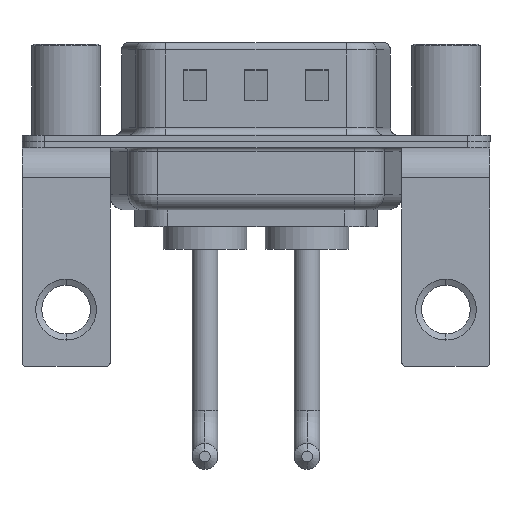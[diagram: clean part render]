
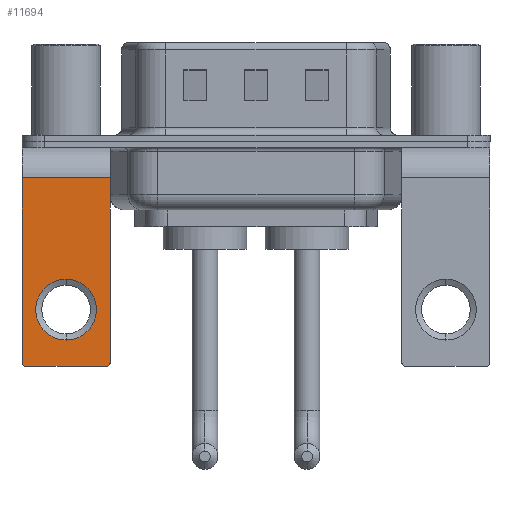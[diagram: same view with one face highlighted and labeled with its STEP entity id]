
A CAD part, front view. The second image highlights one B-rep face of the part: STEP entity #11694.
In plain terms, the highlighted planar face has unit normal (0, -1, 0).
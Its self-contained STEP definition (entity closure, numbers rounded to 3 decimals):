
#491 = EDGE_LOOP ( 'NONE', ( #12679, #11862, #15501, #12673, #6525, #12632 ) ) ;
#604 = EDGE_CURVE ( 'NONE', #1307, #2217, #11024, .T. ) ;
#1099 = CARTESIAN_POINT ( 'NONE',  ( 2.9, -6.25, -2.4 ) ) ;
#1121 = CARTESIAN_POINT ( 'NONE',  ( 0., -6.25, -9.07 ) ) ;
#1208 = VERTEX_POINT ( 'NONE', #5737 ) ;
#1215 = VECTOR ( 'NONE', #6323, 1000. ) ;
#1307 = VERTEX_POINT ( 'NONE', #8716 ) ;
#1532 = ORIENTED_EDGE ( 'NONE', *, *, #15060, .T. ) ;
#2217 = VERTEX_POINT ( 'NONE', #11225 ) ;
#2307 = DIRECTION ( 'NONE',  ( 0., -1., 0. ) ) ;
#2716 = CARTESIAN_POINT ( 'NONE',  ( -2.65, -6.25, -14.8 ) ) ;
#2738 = DIRECTION ( 'NONE',  ( 0., 0., -1. ) ) ;
#2911 = DIRECTION ( 'NONE',  ( 0., 1., 0. ) ) ;
#3023 = EDGE_CURVE ( 'NONE', #14362, #9159, #6748, .T. ) ;
#3037 = ORIENTED_EDGE ( 'NONE', *, *, #14663, .T. ) ;
#3417 = VERTEX_POINT ( 'NONE', #1099 ) ;
#4305 = VERTEX_POINT ( 'NONE', #1121 ) ;
#4631 = LINE ( 'NONE', #9841, #15808 ) ;
#4887 = DIRECTION ( 'NONE',  ( -1., 0., 0. ) ) ;
#4995 = EDGE_LOOP ( 'NONE', ( #1532, #3037 ) ) ;
#5540 = FACE_BOUND ( 'NONE', #4995, .T. ) ;
#5556 = DIRECTION ( 'NONE',  ( 0., 0., 1. ) ) ;
#5737 = CARTESIAN_POINT ( 'NONE',  ( 0., -6.25, -13.07 ) ) ;
#5770 = CARTESIAN_POINT ( 'NONE',  ( -2.9, -6.25, -14.55 ) ) ;
#5901 = CIRCLE ( 'NONE', #15966, 0.25 ) ;
#6263 = CARTESIAN_POINT ( 'NONE',  ( 2.9, -6.25, -2.4 ) ) ;
#6323 = DIRECTION ( 'NONE',  ( 0., 0., -1. ) ) ;
#6525 = ORIENTED_EDGE ( 'NONE', *, *, #15311, .F. ) ;
#6748 = LINE ( 'NONE', #10497, #16271 ) ;
#6910 = EDGE_CURVE ( 'NONE', #1307, #8998, #4631, .T. ) ;
#7039 = DIRECTION ( 'NONE',  ( -1., 0., 0. ) ) ;
#7084 = DIRECTION ( 'NONE',  ( 0., 0., 1. ) ) ;
#7998 = LINE ( 'NONE', #6263, #12092 ) ;
#8716 = CARTESIAN_POINT ( 'NONE',  ( 2.65, -6.25, -14.8 ) ) ;
#8728 = DIRECTION ( 'NONE',  ( 0., 0., 1. ) ) ;
#8998 = VERTEX_POINT ( 'NONE', #2716 ) ;
#9159 = VERTEX_POINT ( 'NONE', #5770 ) ;
#9306 = CARTESIAN_POINT ( 'NONE',  ( 0., -6.25, -11.07 ) ) ;
#9467 = DIRECTION ( 'NONE',  ( 0., 1., 0. ) ) ;
#9841 = CARTESIAN_POINT ( 'NONE',  ( 2.9, -6.25, -14.8 ) ) ;
#10257 = AXIS2_PLACEMENT_3D ( 'NONE', #9306, #2911, #5556 ) ;
#10497 = CARTESIAN_POINT ( 'NONE',  ( -2.9, -6.25, -2.4 ) ) ;
#10552 = CARTESIAN_POINT ( 'NONE',  ( 2.65, -6.25, -14.55 ) ) ;
#10735 = FACE_OUTER_BOUND ( 'NONE', #491, .T. ) ;
#10752 = AXIS2_PLACEMENT_3D ( 'NONE', #10552, #11033, #14782 ) ;
#11024 = CIRCLE ( 'NONE', #10752, 0.25 ) ;
#11033 = DIRECTION ( 'NONE',  ( 0., -1., 0. ) ) ;
#11225 = CARTESIAN_POINT ( 'NONE',  ( 2.9, -6.25, -14.55 ) ) ;
#11264 = CARTESIAN_POINT ( 'NONE',  ( -2.65, -6.25, -14.55 ) ) ;
#11368 = CARTESIAN_POINT ( 'NONE',  ( 0., -6.25, -11.07 ) ) ;
#11594 = CIRCLE ( 'NONE', #14583, 2. ) ;
#11694 = ADVANCED_FACE ( 'NONE', ( #5540, #10735 ), #14824, .F. ) ;
#11862 = ORIENTED_EDGE ( 'NONE', *, *, #16680, .T. ) ;
#12092 = VECTOR ( 'NONE', #4887, 1000. ) ;
#12632 = ORIENTED_EDGE ( 'NONE', *, *, #13301, .T. ) ;
#12673 = ORIENTED_EDGE ( 'NONE', *, *, #604, .T. ) ;
#12679 = ORIENTED_EDGE ( 'NONE', *, *, #3023, .T. ) ;
#12712 = LINE ( 'NONE', #15274, #1215 ) ;
#13221 = CIRCLE ( 'NONE', #10257, 2. ) ;
#13301 = EDGE_CURVE ( 'NONE', #3417, #14362, #7998, .T. ) ;
#13317 = CARTESIAN_POINT ( 'NONE',  ( -2.9, -6.25, -2.4 ) ) ;
#13416 = AXIS2_PLACEMENT_3D ( 'NONE', #15939, #9467, #7084 ) ;
#14362 = VERTEX_POINT ( 'NONE', #13317 ) ;
#14583 = AXIS2_PLACEMENT_3D ( 'NONE', #11368, #16582, #8728 ) ;
#14663 = EDGE_CURVE ( 'NONE', #4305, #1208, #11594, .T. ) ;
#14782 = DIRECTION ( 'NONE',  ( 0., 0., 1. ) ) ;
#14824 = PLANE ( 'NONE',  #13416 ) ;
#15060 = EDGE_CURVE ( 'NONE', #1208, #4305, #13221, .T. ) ;
#15274 = CARTESIAN_POINT ( 'NONE',  ( 2.9, -6.25, -2.4 ) ) ;
#15311 = EDGE_CURVE ( 'NONE', #3417, #2217, #12712, .T. ) ;
#15358 = DIRECTION ( 'NONE',  ( 0., 0., 1. ) ) ;
#15501 = ORIENTED_EDGE ( 'NONE', *, *, #6910, .F. ) ;
#15808 = VECTOR ( 'NONE', #7039, 1000. ) ;
#15939 = CARTESIAN_POINT ( 'NONE',  ( 2.9, -6.25, -2.4 ) ) ;
#15966 = AXIS2_PLACEMENT_3D ( 'NONE', #11264, #2307, #15358 ) ;
#16271 = VECTOR ( 'NONE', #2738, 1000. ) ;
#16582 = DIRECTION ( 'NONE',  ( 0., 1., 0. ) ) ;
#16680 = EDGE_CURVE ( 'NONE', #9159, #8998, #5901, .T. ) ;
